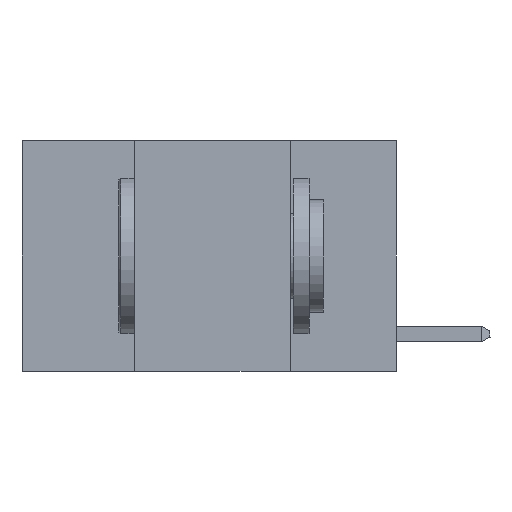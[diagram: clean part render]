
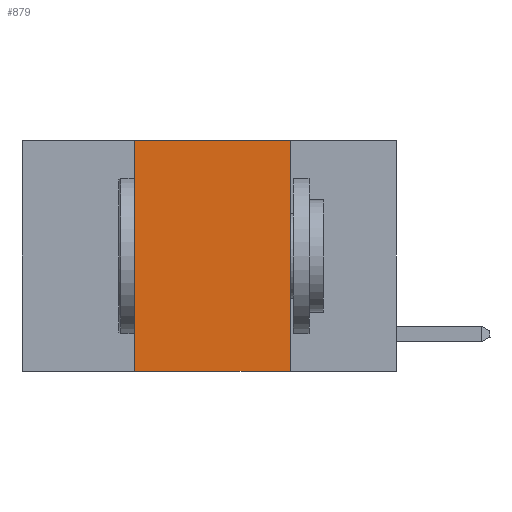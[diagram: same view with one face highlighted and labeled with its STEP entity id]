
A CAD part, left-side view. The second image highlights one B-rep face of the part: STEP entity #879.
In plain terms, the highlighted planar face has unit normal (-1, 0, 0).
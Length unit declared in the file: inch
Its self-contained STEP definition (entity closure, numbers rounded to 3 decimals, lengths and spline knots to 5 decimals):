
#200 = VECTOR ( 'NONE', #18234, 39.37008 ) ;
#346 = CARTESIAN_POINT ( 'NONE',  ( 0., 0.17, 0. ) ) ;
#879 = ADVANCED_FACE ( 'NONE', ( #12198 ), #18404, .F. ) ;
#974 = CARTESIAN_POINT ( 'NONE',  ( 0., 0.6, -0.37 ) ) ;
#1425 = LINE ( 'NONE', #23531, #17585 ) ;
#1896 = VERTEX_POINT ( 'NONE', #22470 ) ;
#4525 = ORIENTED_EDGE ( 'NONE', *, *, #23234, .F. ) ;
#5929 = DIRECTION ( 'NONE',  ( 0., 0., -1. ) ) ;
#6093 = VERTEX_POINT ( 'NONE', #9036 ) ;
#6203 = CARTESIAN_POINT ( 'NONE',  ( 0., 0.6, 0. ) ) ;
#7470 = EDGE_CURVE ( 'NONE', #26221, #1896, #1425, .T. ) ;
#7658 = EDGE_CURVE ( 'NONE', #8254, #6093, #21845, .T. ) ;
#8254 = VERTEX_POINT ( 'NONE', #24492 ) ;
#8982 = LINE ( 'NONE', #974, #20688 ) ;
#9036 = CARTESIAN_POINT ( 'NONE',  ( 0., 0.42, 0. ) ) ;
#10634 = EDGE_LOOP ( 'NONE', ( #22724, #4525, #11822, #14568 ) ) ;
#11586 = CARTESIAN_POINT ( 'NONE',  ( 0., 0.6, 0. ) ) ;
#11822 = ORIENTED_EDGE ( 'NONE', *, *, #7658, .F. ) ;
#11845 = LINE ( 'NONE', #11586, #16209 ) ;
#12198 = FACE_OUTER_BOUND ( 'NONE', #10634, .T. ) ;
#14568 = ORIENTED_EDGE ( 'NONE', *, *, #16805, .T. ) ;
#16209 = VECTOR ( 'NONE', #21805, 39.37008 ) ;
#16805 = EDGE_CURVE ( 'NONE', #8254, #1896, #8982, .T. ) ;
#17585 = VECTOR ( 'NONE', #21787, 39.37008 ) ;
#18234 = DIRECTION ( 'NONE',  ( 0., 0., 1. ) ) ;
#18404 = PLANE ( 'NONE',  #25833 ) ;
#19041 = DIRECTION ( 'NONE',  ( 0., -1., 0. ) ) ;
#20133 = DIRECTION ( 'NONE',  ( 1., 0., 0. ) ) ;
#20688 = VECTOR ( 'NONE', #19041, 39.37008 ) ;
#21787 = DIRECTION ( 'NONE',  ( 0., 0., -1. ) ) ;
#21805 = DIRECTION ( 'NONE',  ( 0., -1., 0. ) ) ;
#21845 = LINE ( 'NONE', #24261, #200 ) ;
#22470 = CARTESIAN_POINT ( 'NONE',  ( 0., 0.17, -0.37 ) ) ;
#22724 = ORIENTED_EDGE ( 'NONE', *, *, #7470, .F. ) ;
#23234 = EDGE_CURVE ( 'NONE', #6093, #26221, #11845, .T. ) ;
#23531 = CARTESIAN_POINT ( 'NONE',  ( 0., 0.17, 0. ) ) ;
#24261 = CARTESIAN_POINT ( 'NONE',  ( 0., 0.42, 0. ) ) ;
#24492 = CARTESIAN_POINT ( 'NONE',  ( 0., 0.42, -0.37 ) ) ;
#25833 = AXIS2_PLACEMENT_3D ( 'NONE', #6203, #20133, #5929 ) ;
#26221 = VERTEX_POINT ( 'NONE', #346 ) ;
